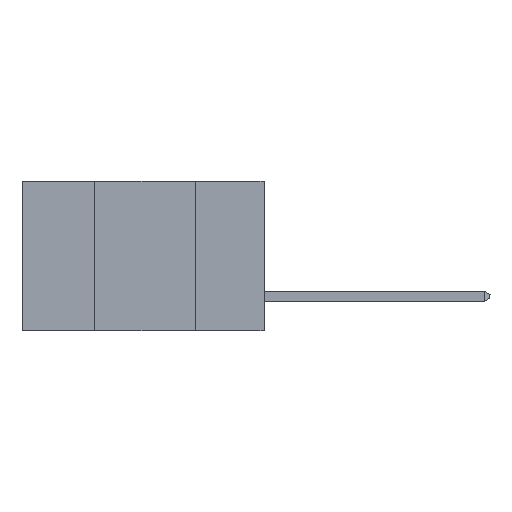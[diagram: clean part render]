
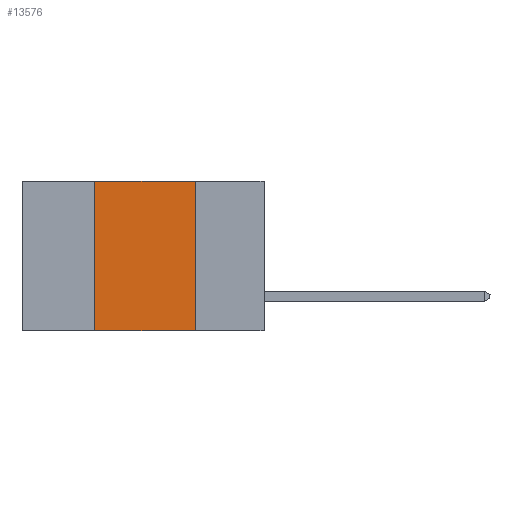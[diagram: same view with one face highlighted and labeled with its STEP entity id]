
A CAD part, left-side view. The second image highlights one B-rep face of the part: STEP entity #13576.
In plain terms, the highlighted planar face has unit normal (-1, 0, 0).
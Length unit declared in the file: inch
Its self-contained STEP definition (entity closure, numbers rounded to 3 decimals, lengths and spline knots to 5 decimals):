
#235 = ORIENTED_EDGE ( 'NONE', *, *, #5119, .F. ) ;
#494 = LINE ( 'NONE', #12429, #4526 ) ;
#1132 = LINE ( 'NONE', #10371, #11203 ) ;
#1674 = LINE ( 'NONE', #15053, #2789 ) ;
#1732 = DIRECTION ( 'NONE',  ( 0., 0., -1. ) ) ;
#2245 = ORIENTED_EDGE ( 'NONE', *, *, #4540, .T. ) ;
#2599 = DIRECTION ( 'NONE',  ( 0., -1., 0. ) ) ;
#2789 = VECTOR ( 'NONE', #11209, 39.37008 ) ;
#3878 = VERTEX_POINT ( 'NONE', #14766 ) ;
#4087 = CARTESIAN_POINT ( 'NONE',  ( 0., 0.6, 0. ) ) ;
#4457 = DIRECTION ( 'NONE',  ( 0., 0., 1. ) ) ;
#4526 = VECTOR ( 'NONE', #1732, 39.37008 ) ;
#4540 = EDGE_CURVE ( 'NONE', #3878, #11614, #9705, .T. ) ;
#4892 = ORIENTED_EDGE ( 'NONE', *, *, #14996, .F. ) ;
#4971 = EDGE_LOOP ( 'NONE', ( #235, #13427, #4892, #2245 ) ) ;
#5119 = EDGE_CURVE ( 'NONE', #10980, #11614, #494, .T. ) ;
#5124 = VERTEX_POINT ( 'NONE', #11262 ) ;
#6752 = AXIS2_PLACEMENT_3D ( 'NONE', #4087, #12583, #8891 ) ;
#7100 = CARTESIAN_POINT ( 'NONE',  ( 0., 0.17, -0.37 ) ) ;
#7240 = VECTOR ( 'NONE', #2599, 39.37008 ) ;
#7336 = EDGE_CURVE ( 'NONE', #5124, #10980, #1674, .T. ) ;
#7519 = CARTESIAN_POINT ( 'NONE',  ( 0., 0.17, 0. ) ) ;
#8891 = DIRECTION ( 'NONE',  ( 0., 0., -1. ) ) ;
#9705 = LINE ( 'NONE', #13160, #7240 ) ;
#10371 = CARTESIAN_POINT ( 'NONE',  ( 0., 0.42, -0.37 ) ) ;
#10980 = VERTEX_POINT ( 'NONE', #7519 ) ;
#11203 = VECTOR ( 'NONE', #4457, 39.37008 ) ;
#11209 = DIRECTION ( 'NONE',  ( 0., -1., 0. ) ) ;
#11262 = CARTESIAN_POINT ( 'NONE',  ( 0., 0.42, 0. ) ) ;
#11614 = VERTEX_POINT ( 'NONE', #7100 ) ;
#12429 = CARTESIAN_POINT ( 'NONE',  ( 0., 0.17, -0.37 ) ) ;
#12583 = DIRECTION ( 'NONE',  ( 1., 0., 0. ) ) ;
#13160 = CARTESIAN_POINT ( 'NONE',  ( 0., 0.6, -0.37 ) ) ;
#13427 = ORIENTED_EDGE ( 'NONE', *, *, #7336, .F. ) ;
#13537 = PLANE ( 'NONE',  #6752 ) ;
#13576 = ADVANCED_FACE ( 'NONE', ( #13849 ), #13537, .F. ) ;
#13849 = FACE_OUTER_BOUND ( 'NONE', #4971, .T. ) ;
#14766 = CARTESIAN_POINT ( 'NONE',  ( 0., 0.42, -0.37 ) ) ;
#14996 = EDGE_CURVE ( 'NONE', #3878, #5124, #1132, .T. ) ;
#15053 = CARTESIAN_POINT ( 'NONE',  ( 0., 0.6, 0. ) ) ;
